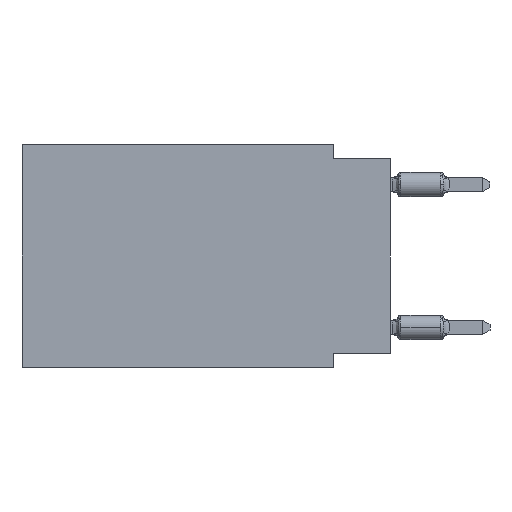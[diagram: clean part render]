
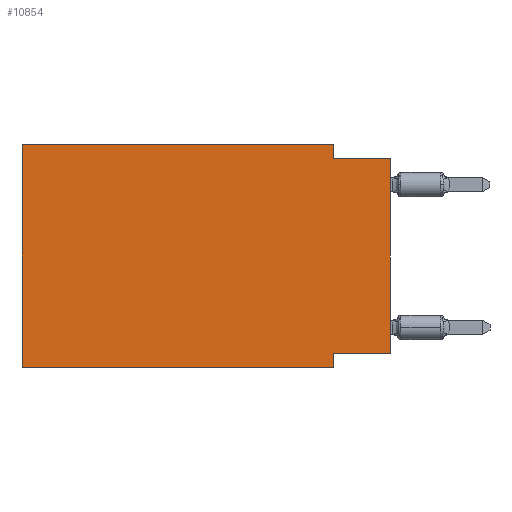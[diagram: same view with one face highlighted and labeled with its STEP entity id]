
A CAD part, left-side view. The second image highlights one B-rep face of the part: STEP entity #10854.
In plain terms, the highlighted planar face has unit normal (-1, 0, 0).
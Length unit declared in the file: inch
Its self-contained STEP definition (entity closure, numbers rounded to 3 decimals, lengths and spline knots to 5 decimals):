
#9 = EDGE_CURVE ( 'NONE', #11751, #7091, #7325, .T. ) ;
#15 = CARTESIAN_POINT ( 'NONE',  ( 0., 0., 0. ) ) ;
#156 = VECTOR ( 'NONE', #4771, 39.37008 ) ;
#245 = LINE ( 'NONE', #6023, #14350 ) ;
#944 = VECTOR ( 'NONE', #1343, 39.37008 ) ;
#1098 = VERTEX_POINT ( 'NONE', #17227 ) ;
#1146 = CARTESIAN_POINT ( 'NONE',  ( 0., 0.645, 0. ) ) ;
#1148 = EDGE_CURVE ( 'NONE', #16292, #12646, #13067, .T. ) ;
#1252 = VERTEX_POINT ( 'NONE', #4787 ) ;
#1279 = VERTEX_POINT ( 'NONE', #14971 ) ;
#1343 = DIRECTION ( 'NONE',  ( 0., -1., 0. ) ) ;
#1503 = ORIENTED_EDGE ( 'NONE', *, *, #12835, .F. ) ;
#1660 = PLANE ( 'NONE',  #6892 ) ;
#1933 = CARTESIAN_POINT ( 'NONE',  ( 0., 0., -0.025 ) ) ;
#2121 = VECTOR ( 'NONE', #12967, 39.37008 ) ;
#2743 = CARTESIAN_POINT ( 'NONE',  ( 0., 0.1, -0.39 ) ) ;
#2823 = LINE ( 'NONE', #10218, #11490 ) ;
#2851 = EDGE_LOOP ( 'NONE', ( #6024, #11372, #5401, #9532, #15548, #16769, #1503, #12273 ) ) ;
#3075 = DIRECTION ( 'NONE',  ( 0., 0., 1. ) ) ;
#3172 = DIRECTION ( 'NONE',  ( 0., 0., -1. ) ) ;
#3227 = EDGE_CURVE ( 'NONE', #12646, #9745, #15484, .T. ) ;
#3863 = CARTESIAN_POINT ( 'NONE',  ( 0., 0.1, 0. ) ) ;
#3955 = EDGE_CURVE ( 'NONE', #1279, #7091, #245, .T. ) ;
#4771 = DIRECTION ( 'NONE',  ( 0., 1., 0. ) ) ;
#4787 = CARTESIAN_POINT ( 'NONE',  ( 0., 0.1, -0.39 ) ) ;
#5401 = ORIENTED_EDGE ( 'NONE', *, *, #14529, .F. ) ;
#5485 = EDGE_CURVE ( 'NONE', #11751, #1098, #13155, .T. ) ;
#5643 = CARTESIAN_POINT ( 'NONE',  ( 0., 0.645, 0. ) ) ;
#6023 = CARTESIAN_POINT ( 'NONE',  ( 0., 0., -0.025 ) ) ;
#6024 = ORIENTED_EDGE ( 'NONE', *, *, #9, .T. ) ;
#6892 = AXIS2_PLACEMENT_3D ( 'NONE', #9040, #14662, #3172 ) ;
#7091 = VERTEX_POINT ( 'NONE', #1933 ) ;
#7281 = DIRECTION ( 'NONE',  ( 0., 0., -1. ) ) ;
#7325 = LINE ( 'NONE', #15, #16591 ) ;
#7935 = CARTESIAN_POINT ( 'NONE',  ( 0., 0.645, -0.39 ) ) ;
#8035 = LINE ( 'NONE', #7935, #16222 ) ;
#9002 = EDGE_CURVE ( 'NONE', #16292, #1252, #8035, .T. ) ;
#9040 = CARTESIAN_POINT ( 'NONE',  ( 0., 0.645, 0. ) ) ;
#9490 = CARTESIAN_POINT ( 'NONE',  ( 0., 0.645, 0. ) ) ;
#9532 = ORIENTED_EDGE ( 'NONE', *, *, #3227, .F. ) ;
#9676 = VECTOR ( 'NONE', #7281, 39.37008 ) ;
#9745 = VERTEX_POINT ( 'NONE', #3863 ) ;
#10218 = CARTESIAN_POINT ( 'NONE',  ( 0., 0.1, 0. ) ) ;
#10854 = ADVANCED_FACE ( 'NONE', ( #16161 ), #1660, .F. ) ;
#11372 = ORIENTED_EDGE ( 'NONE', *, *, #3955, .F. ) ;
#11490 = VECTOR ( 'NONE', #18745, 39.37008 ) ;
#11751 = VERTEX_POINT ( 'NONE', #15735 ) ;
#11828 = DIRECTION ( 'NONE',  ( 0., -1., 0. ) ) ;
#12210 = CARTESIAN_POINT ( 'NONE',  ( 0., 0.645, -0.39 ) ) ;
#12273 = ORIENTED_EDGE ( 'NONE', *, *, #5485, .F. ) ;
#12646 = VERTEX_POINT ( 'NONE', #9490 ) ;
#12835 = EDGE_CURVE ( 'NONE', #1098, #1252, #12895, .T. ) ;
#12895 = LINE ( 'NONE', #2743, #9676 ) ;
#12967 = DIRECTION ( 'NONE',  ( 0., 0., 1. ) ) ;
#13067 = LINE ( 'NONE', #5643, #2121 ) ;
#13155 = LINE ( 'NONE', #17780, #156 ) ;
#14350 = VECTOR ( 'NONE', #11828, 39.37008 ) ;
#14529 = EDGE_CURVE ( 'NONE', #9745, #1279, #2823, .T. ) ;
#14662 = DIRECTION ( 'NONE',  ( 1., 0., 0. ) ) ;
#14971 = CARTESIAN_POINT ( 'NONE',  ( 0., 0.1, -0.025 ) ) ;
#15484 = LINE ( 'NONE', #1146, #944 ) ;
#15548 = ORIENTED_EDGE ( 'NONE', *, *, #1148, .F. ) ;
#15735 = CARTESIAN_POINT ( 'NONE',  ( 0., 0., -0.365 ) ) ;
#16161 = FACE_OUTER_BOUND ( 'NONE', #2851, .T. ) ;
#16222 = VECTOR ( 'NONE', #18089, 39.37008 ) ;
#16292 = VERTEX_POINT ( 'NONE', #12210 ) ;
#16591 = VECTOR ( 'NONE', #3075, 39.37008 ) ;
#16769 = ORIENTED_EDGE ( 'NONE', *, *, #9002, .T. ) ;
#17227 = CARTESIAN_POINT ( 'NONE',  ( 0., 0.1, -0.365 ) ) ;
#17780 = CARTESIAN_POINT ( 'NONE',  ( 0., 0., -0.365 ) ) ;
#18089 = DIRECTION ( 'NONE',  ( 0., -1., 0. ) ) ;
#18745 = DIRECTION ( 'NONE',  ( 0., 0., -1. ) ) ;
